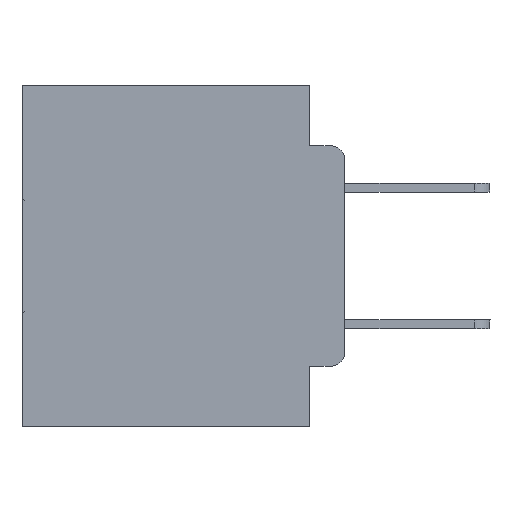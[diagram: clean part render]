
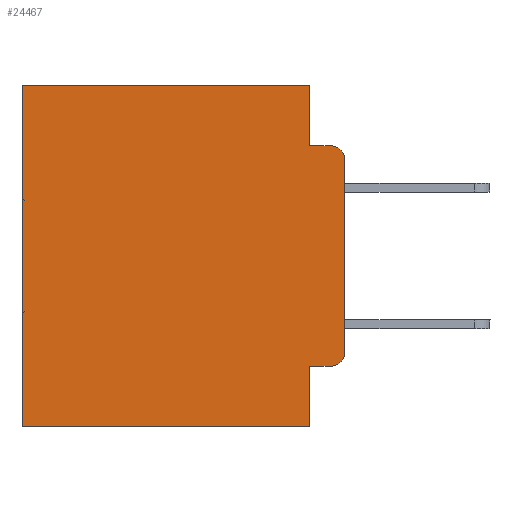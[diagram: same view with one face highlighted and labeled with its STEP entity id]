
A CAD part, left-side view. The second image highlights one B-rep face of the part: STEP entity #24467.
In plain terms, the highlighted planar face has unit normal (-1, 0, 0).
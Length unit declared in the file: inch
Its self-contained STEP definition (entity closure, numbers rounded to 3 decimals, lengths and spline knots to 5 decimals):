
#289 = ORIENTED_EDGE ( 'NONE', *, *, #7780, .T. ) ;
#845 = CARTESIAN_POINT ( 'NONE',  ( 0.298, 0.473, 0. ) ) ;
#2217 = DIRECTION ( 'NONE',  ( 0., 0., -1. ) ) ;
#2543 = DIRECTION ( 'NONE',  ( 0., 1., 0. ) ) ;
#2866 = VECTOR ( 'NONE', #32572, 39.37008 ) ;
#3118 = CARTESIAN_POINT ( 'NONE',  ( 0.298, 0.051, 0. ) ) ;
#3473 = CARTESIAN_POINT ( 'NONE',  ( 0.298, 0.02, -0.4115 ) ) ;
#4168 = LINE ( 'NONE', #22659, #4583 ) ;
#4583 = VECTOR ( 'NONE', #25232, 39.37008 ) ;
#4586 = EDGE_CURVE ( 'NONE', #12468, #5565, #18979, .T. ) ;
#5565 = VERTEX_POINT ( 'NONE', #25474 ) ;
#6371 = DIRECTION ( 'NONE',  ( 0., -1., 0. ) ) ;
#6858 = EDGE_CURVE ( 'NONE', #14905, #26977, #14813, .T. ) ;
#7623 = DIRECTION ( 'NONE',  ( 1., 0., 0. ) ) ;
#7735 = EDGE_LOOP ( 'NONE', ( #25791, #7885, #24323, #25974, #33182, #8408, #9414, #19760, #289, #24848 ) ) ;
#7780 = EDGE_CURVE ( 'NONE', #12468, #19221, #20127, .T. ) ;
#7885 = ORIENTED_EDGE ( 'NONE', *, *, #24039, .T. ) ;
#8408 = ORIENTED_EDGE ( 'NONE', *, *, #15353, .T. ) ;
#8653 = DIRECTION ( 'NONE',  ( 0., 0., -1. ) ) ;
#9414 = ORIENTED_EDGE ( 'NONE', *, *, #19280, .F. ) ;
#9700 = VECTOR ( 'NONE', #18569, 39.37008 ) ;
#10200 = LINE ( 'NONE', #3118, #24608 ) ;
#10361 = AXIS2_PLACEMENT_3D ( 'NONE', #30790, #7623, #2217 ) ;
#10578 = CARTESIAN_POINT ( 'NONE',  ( 0.298, 0.02, -0.3915 ) ) ;
#11003 = DIRECTION ( 'NONE',  ( -1., 0., 0. ) ) ;
#11289 = CARTESIAN_POINT ( 'NONE',  ( 0.298, 0.051, -0.0885 ) ) ;
#11483 = LINE ( 'NONE', #11289, #31101 ) ;
#12468 = VERTEX_POINT ( 'NONE', #24072 ) ;
#12631 = VERTEX_POINT ( 'NONE', #26837 ) ;
#12719 = DIRECTION ( 'NONE',  ( -1., 0., 0. ) ) ;
#13439 = EDGE_CURVE ( 'NONE', #14905, #14343, #10200, .T. ) ;
#14343 = VERTEX_POINT ( 'NONE', #27086 ) ;
#14813 = LINE ( 'NONE', #28101, #30854 ) ;
#14905 = VERTEX_POINT ( 'NONE', #16730 ) ;
#15353 = EDGE_CURVE ( 'NONE', #26977, #12631, #16540, .T. ) ;
#15747 = VERTEX_POINT ( 'NONE', #19264 ) ;
#16251 = LINE ( 'NONE', #32403, #33107 ) ;
#16540 = LINE ( 'NONE', #17573, #2866 ) ;
#16730 = CARTESIAN_POINT ( 'NONE',  ( 0.298, 0.051, 0. ) ) ;
#17070 = DIRECTION ( 'NONE',  ( 0., 1., 0. ) ) ;
#17367 = VECTOR ( 'NONE', #23308, 39.37008 ) ;
#17573 = CARTESIAN_POINT ( 'NONE',  ( 0.298, 0.473, 0. ) ) ;
#17658 = VERTEX_POINT ( 'NONE', #21472 ) ;
#18569 = DIRECTION ( 'NONE',  ( 0., -1., 0. ) ) ;
#18979 = LINE ( 'NONE', #31035, #17367 ) ;
#19159 = CIRCLE ( 'NONE', #26858, 0.02 ) ;
#19221 = VERTEX_POINT ( 'NONE', #3473 ) ;
#19264 = CARTESIAN_POINT ( 'NONE',  ( 0.298, 0., -0.1085 ) ) ;
#19280 = EDGE_CURVE ( 'NONE', #5565, #12631, #16251, .T. ) ;
#19760 = ORIENTED_EDGE ( 'NONE', *, *, #4586, .F. ) ;
#20127 = LINE ( 'NONE', #21485, #9700 ) ;
#20538 = VERTEX_POINT ( 'NONE', #27525 ) ;
#21472 = CARTESIAN_POINT ( 'NONE',  ( 0.298, 0.02, -0.0885 ) ) ;
#21485 = CARTESIAN_POINT ( 'NONE',  ( 0.298, 0.051, -0.4115 ) ) ;
#22659 = CARTESIAN_POINT ( 'NONE',  ( 0.298, 0., 0. ) ) ;
#22892 = EDGE_CURVE ( 'NONE', #19221, #20538, #32083, .T. ) ;
#23308 = DIRECTION ( 'NONE',  ( 0., 0., -1. ) ) ;
#24039 = EDGE_CURVE ( 'NONE', #15747, #17658, #19159, .T. ) ;
#24072 = CARTESIAN_POINT ( 'NONE',  ( 0.298, 0.051, -0.4115 ) ) ;
#24323 = ORIENTED_EDGE ( 'NONE', *, *, #31468, .F. ) ;
#24467 = ADVANCED_FACE ( 'NONE', ( #27128 ), #27768, .F. ) ;
#24608 = VECTOR ( 'NONE', #26565, 39.37008 ) ;
#24848 = ORIENTED_EDGE ( 'NONE', *, *, #22892, .T. ) ;
#25232 = DIRECTION ( 'NONE',  ( 0., 0., -1. ) ) ;
#25474 = CARTESIAN_POINT ( 'NONE',  ( 0.298, 0.051, -0.5 ) ) ;
#25791 = ORIENTED_EDGE ( 'NONE', *, *, #32749, .F. ) ;
#25971 = AXIS2_PLACEMENT_3D ( 'NONE', #10578, #12719, #30515 ) ;
#25974 = ORIENTED_EDGE ( 'NONE', *, *, #13439, .F. ) ;
#26565 = DIRECTION ( 'NONE',  ( 0., 0., -1. ) ) ;
#26837 = CARTESIAN_POINT ( 'NONE',  ( 0.298, 0.473, -0.5 ) ) ;
#26858 = AXIS2_PLACEMENT_3D ( 'NONE', #31271, #11003, #8653 ) ;
#26977 = VERTEX_POINT ( 'NONE', #845 ) ;
#27086 = CARTESIAN_POINT ( 'NONE',  ( 0.298, 0.051, -0.0885 ) ) ;
#27128 = FACE_OUTER_BOUND ( 'NONE', #7735, .T. ) ;
#27525 = CARTESIAN_POINT ( 'NONE',  ( 0.298, 0., -0.3915 ) ) ;
#27768 = PLANE ( 'NONE',  #10361 ) ;
#28101 = CARTESIAN_POINT ( 'NONE',  ( 0.298, 0., 0. ) ) ;
#30515 = DIRECTION ( 'NONE',  ( 0., 0., -1. ) ) ;
#30790 = CARTESIAN_POINT ( 'NONE',  ( 0.298, 0., 0. ) ) ;
#30854 = VECTOR ( 'NONE', #2543, 39.37008 ) ;
#31035 = CARTESIAN_POINT ( 'NONE',  ( 0.298, 0.051, 0. ) ) ;
#31101 = VECTOR ( 'NONE', #6371, 39.37008 ) ;
#31271 = CARTESIAN_POINT ( 'NONE',  ( 0.298, 0.02, -0.1085 ) ) ;
#31468 = EDGE_CURVE ( 'NONE', #14343, #17658, #11483, .T. ) ;
#32083 = CIRCLE ( 'NONE', #25971, 0.02 ) ;
#32403 = CARTESIAN_POINT ( 'NONE',  ( 0.298, 0., -0.5 ) ) ;
#32572 = DIRECTION ( 'NONE',  ( 0., 0., -1. ) ) ;
#32749 = EDGE_CURVE ( 'NONE', #15747, #20538, #4168, .T. ) ;
#33107 = VECTOR ( 'NONE', #17070, 39.37008 ) ;
#33182 = ORIENTED_EDGE ( 'NONE', *, *, #6858, .T. ) ;
